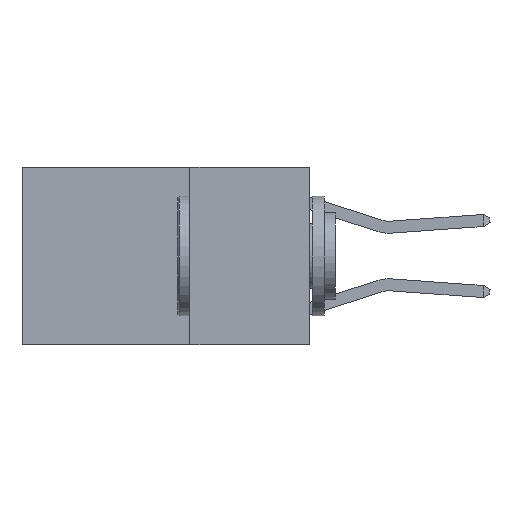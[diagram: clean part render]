
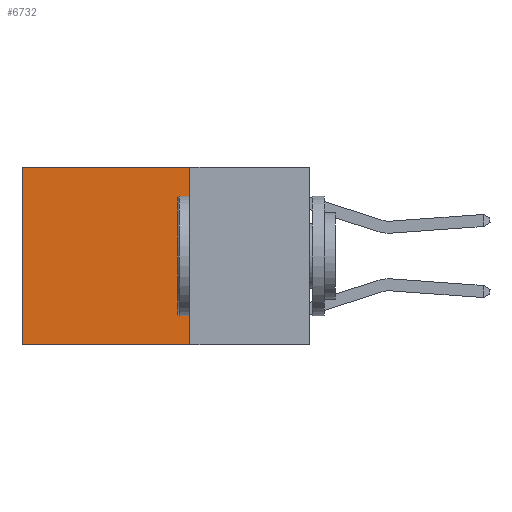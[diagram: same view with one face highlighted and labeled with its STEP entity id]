
A CAD part, left-side view. The second image highlights one B-rep face of the part: STEP entity #6732.
In plain terms, the highlighted planar face has unit normal (-1, 0, 0).
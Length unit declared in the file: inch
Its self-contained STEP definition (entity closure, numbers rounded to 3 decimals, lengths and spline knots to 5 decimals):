
#474 = CARTESIAN_POINT ( 'NONE',  ( 0.2625, 0.6, 0. ) ) ;
#501 = LINE ( 'NONE', #4612, #3122 ) ;
#546 = LINE ( 'NONE', #8892, #7215 ) ;
#561 = DIRECTION ( 'NONE',  ( 0., 1., 0. ) ) ;
#693 = EDGE_CURVE ( 'NONE', #6893, #12843, #9965, .T. ) ;
#2452 = EDGE_LOOP ( 'NONE', ( #3617, #6682, #8306, #9780 ) ) ;
#3122 = VECTOR ( 'NONE', #561, 39.37008 ) ;
#3361 = CARTESIAN_POINT ( 'NONE',  ( 0.2625, 0.25, 0. ) ) ;
#3425 = DIRECTION ( 'NONE',  ( 0., 0., -1. ) ) ;
#3617 = ORIENTED_EDGE ( 'NONE', *, *, #693, .T. ) ;
#3708 = DIRECTION ( 'NONE',  ( 0., 0., -1. ) ) ;
#4056 = EDGE_CURVE ( 'NONE', #6069, #6160, #10812, .T. ) ;
#4496 = CARTESIAN_POINT ( 'NONE',  ( 0.2625, 0.25, 0. ) ) ;
#4612 = CARTESIAN_POINT ( 'NONE',  ( 0.2625, 0.25, -0.37 ) ) ;
#5198 = FACE_OUTER_BOUND ( 'NONE', #2452, .T. ) ;
#5270 = PLANE ( 'NONE',  #5569 ) ;
#5569 = AXIS2_PLACEMENT_3D ( 'NONE', #12756, #11688, #12566 ) ;
#5811 = DIRECTION ( 'NONE',  ( 0., 1., 0. ) ) ;
#6069 = VERTEX_POINT ( 'NONE', #4496 ) ;
#6160 = VERTEX_POINT ( 'NONE', #13328 ) ;
#6682 = ORIENTED_EDGE ( 'NONE', *, *, #10224, .F. ) ;
#6732 = ADVANCED_FACE ( 'NONE', ( #5198 ), #5270, .F. ) ;
#6893 = VERTEX_POINT ( 'NONE', #474 ) ;
#7148 = CARTESIAN_POINT ( 'NONE',  ( 0.2625, 0.6, -0.37 ) ) ;
#7215 = VECTOR ( 'NONE', #5811, 39.37008 ) ;
#8306 = ORIENTED_EDGE ( 'NONE', *, *, #4056, .F. ) ;
#8684 = VECTOR ( 'NONE', #3708, 39.37008 ) ;
#8892 = CARTESIAN_POINT ( 'NONE',  ( 0.2625, 0.25, 0. ) ) ;
#9780 = ORIENTED_EDGE ( 'NONE', *, *, #10680, .T. ) ;
#9965 = LINE ( 'NONE', #13181, #8684 ) ;
#10224 = EDGE_CURVE ( 'NONE', #6160, #12843, #501, .T. ) ;
#10680 = EDGE_CURVE ( 'NONE', #6069, #6893, #546, .T. ) ;
#10812 = LINE ( 'NONE', #3361, #12670 ) ;
#11688 = DIRECTION ( 'NONE',  ( 1., 0., 0. ) ) ;
#12566 = DIRECTION ( 'NONE',  ( 0., 0., -1. ) ) ;
#12670 = VECTOR ( 'NONE', #3425, 39.37008 ) ;
#12756 = CARTESIAN_POINT ( 'NONE',  ( 0.2625, 0.25, 0. ) ) ;
#12843 = VERTEX_POINT ( 'NONE', #7148 ) ;
#13181 = CARTESIAN_POINT ( 'NONE',  ( 0.2625, 0.6, 0. ) ) ;
#13328 = CARTESIAN_POINT ( 'NONE',  ( 0.2625, 0.25, -0.37 ) ) ;
